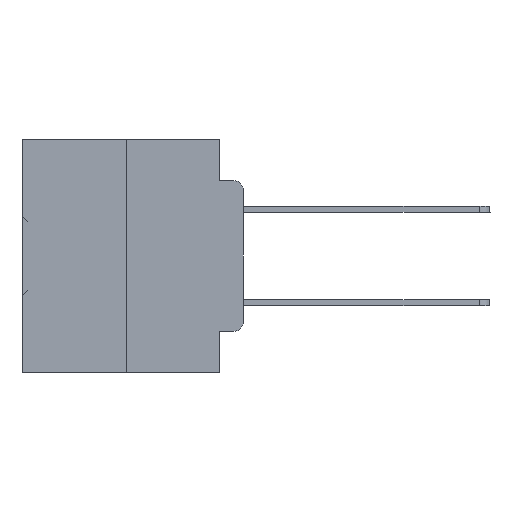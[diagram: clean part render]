
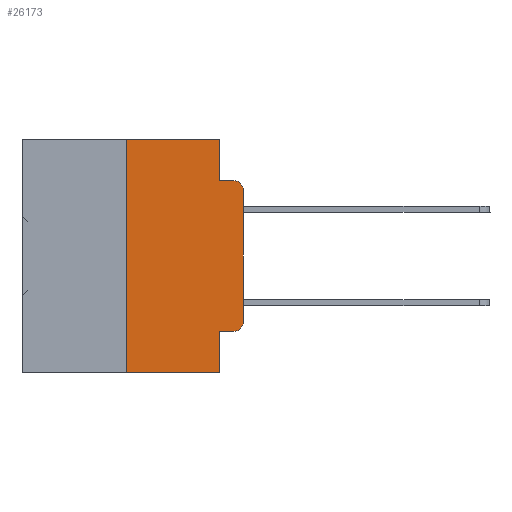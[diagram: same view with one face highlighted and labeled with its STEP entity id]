
A CAD part, left-side view. The second image highlights one B-rep face of the part: STEP entity #26173.
In plain terms, the highlighted planar face has unit normal (-1, 0, 0).
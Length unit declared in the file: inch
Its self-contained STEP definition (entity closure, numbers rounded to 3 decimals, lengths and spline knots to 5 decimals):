
#393 = FACE_OUTER_BOUND ( 'NONE', #2416, .T. ) ;
#561 = LINE ( 'NONE', #35942, #15969 ) ;
#688 = CARTESIAN_POINT ( 'NONE',  ( 0., 0.051, -0.4115 ) ) ;
#721 = EDGE_CURVE ( 'NONE', #11997, #14356, #5320, .T. ) ;
#747 = VERTEX_POINT ( 'NONE', #24021 ) ;
#1299 = DIRECTION ( 'NONE',  ( 0., -1., 0. ) ) ;
#1808 = DIRECTION ( 'NONE',  ( 0., 0., -1. ) ) ;
#2099 = LINE ( 'NONE', #9450, #25305 ) ;
#2406 = LINE ( 'NONE', #12970, #17697 ) ;
#2416 = EDGE_LOOP ( 'NONE', ( #24014, #24961, #5659, #21739, #38669, #31845, #33665, #26746, #3658, #13787 ) ) ;
#2659 = VERTEX_POINT ( 'NONE', #688 ) ;
#3182 = VERTEX_POINT ( 'NONE', #6799 ) ;
#3426 = VERTEX_POINT ( 'NONE', #30335 ) ;
#3658 = ORIENTED_EDGE ( 'NONE', *, *, #20122, .T. ) ;
#3841 = CIRCLE ( 'NONE', #37408, 0.02 ) ;
#4824 = LINE ( 'NONE', #29745, #35655 ) ;
#5126 = DIRECTION ( 'NONE',  ( 1., 0., 0. ) ) ;
#5320 = LINE ( 'NONE', #20551, #29268 ) ;
#5659 = ORIENTED_EDGE ( 'NONE', *, *, #33970, .F. ) ;
#6799 = CARTESIAN_POINT ( 'NONE',  ( 0., 0.25, 0. ) ) ;
#6877 = VERTEX_POINT ( 'NONE', #36498 ) ;
#7035 = CARTESIAN_POINT ( 'NONE',  ( 0., 0., -0.1085 ) ) ;
#7409 = CARTESIAN_POINT ( 'NONE',  ( 0., 0.25, -0.5 ) ) ;
#7493 = CIRCLE ( 'NONE', #21667, 0.02 ) ;
#8132 = LINE ( 'NONE', #19846, #14336 ) ;
#9295 = EDGE_CURVE ( 'NONE', #747, #32645, #2099, .T. ) ;
#9319 = DIRECTION ( 'NONE',  ( 0., 0., 1. ) ) ;
#9450 = CARTESIAN_POINT ( 'NONE',  ( 0., 0., 0. ) ) ;
#10491 = DIRECTION ( 'NONE',  ( 0., -1., 0. ) ) ;
#11108 = DIRECTION ( 'NONE',  ( -1., 0., 0. ) ) ;
#11997 = VERTEX_POINT ( 'NONE', #7409 ) ;
#12260 = VECTOR ( 'NONE', #1299, 39.37008 ) ;
#12970 = CARTESIAN_POINT ( 'NONE',  ( 0., 0.051, 0. ) ) ;
#13787 = ORIENTED_EDGE ( 'NONE', *, *, #18120, .T. ) ;
#14336 = VECTOR ( 'NONE', #22830, 39.37008 ) ;
#14356 = VERTEX_POINT ( 'NONE', #35133 ) ;
#14873 = VERTEX_POINT ( 'NONE', #37246 ) ;
#15969 = VECTOR ( 'NONE', #18272, 39.37008 ) ;
#15975 = DIRECTION ( 'NONE',  ( 0., 0., -1. ) ) ;
#16295 = VECTOR ( 'NONE', #10491, 39.37008 ) ;
#17183 = DIRECTION ( 'NONE',  ( 0., -1., 0. ) ) ;
#17697 = VECTOR ( 'NONE', #15975, 39.37008 ) ;
#18114 = AXIS2_PLACEMENT_3D ( 'NONE', #23183, #5126, #26160 ) ;
#18120 = EDGE_CURVE ( 'NONE', #3426, #747, #3841, .T. ) ;
#18272 = DIRECTION ( 'NONE',  ( 0., 0., 1. ) ) ;
#19080 = VERTEX_POINT ( 'NONE', #29603 ) ;
#19846 = CARTESIAN_POINT ( 'NONE',  ( 0., 0.473, 0. ) ) ;
#20054 = DIRECTION ( 'NONE',  ( -1., 0., 0. ) ) ;
#20122 = EDGE_CURVE ( 'NONE', #2659, #3426, #34964, .T. ) ;
#20551 = CARTESIAN_POINT ( 'NONE',  ( 0., 0.473, -0.5 ) ) ;
#21667 = AXIS2_PLACEMENT_3D ( 'NONE', #37681, #20054, #1808 ) ;
#21739 = ORIENTED_EDGE ( 'NONE', *, *, #32020, .F. ) ;
#22138 = EDGE_CURVE ( 'NONE', #2659, #14356, #4824, .T. ) ;
#22570 = CARTESIAN_POINT ( 'NONE',  ( 0., 0.051, -0.4115 ) ) ;
#22830 = DIRECTION ( 'NONE',  ( 0., -1., 0. ) ) ;
#23183 = CARTESIAN_POINT ( 'NONE',  ( 0., 0.473, 0. ) ) ;
#24014 = ORIENTED_EDGE ( 'NONE', *, *, #9295, .T. ) ;
#24021 = CARTESIAN_POINT ( 'NONE',  ( 0., 0., -0.3915 ) ) ;
#24961 = ORIENTED_EDGE ( 'NONE', *, *, #37881, .T. ) ;
#25305 = VECTOR ( 'NONE', #9319, 39.37008 ) ;
#26160 = DIRECTION ( 'NONE',  ( 0., 0., -1. ) ) ;
#26173 = ADVANCED_FACE ( 'NONE', ( #393 ), #37828, .F. ) ;
#26746 = ORIENTED_EDGE ( 'NONE', *, *, #22138, .F. ) ;
#28918 = CARTESIAN_POINT ( 'NONE',  ( 0., 0.02, -0.3915 ) ) ;
#29268 = VECTOR ( 'NONE', #17183, 39.37008 ) ;
#29271 = LINE ( 'NONE', #31315, #16295 ) ;
#29603 = CARTESIAN_POINT ( 'NONE',  ( 0., 0.051, -0.0885 ) ) ;
#29745 = CARTESIAN_POINT ( 'NONE',  ( 0., 0.051, 0. ) ) ;
#30033 = EDGE_CURVE ( 'NONE', #11997, #3182, #561, .T. ) ;
#30335 = CARTESIAN_POINT ( 'NONE',  ( 0., 0.02, -0.4115 ) ) ;
#31315 = CARTESIAN_POINT ( 'NONE',  ( 0., 0.051, -0.0885 ) ) ;
#31845 = ORIENTED_EDGE ( 'NONE', *, *, #30033, .F. ) ;
#31905 = DIRECTION ( 'NONE',  ( 0., 0., -1. ) ) ;
#32020 = EDGE_CURVE ( 'NONE', #6877, #19080, #2406, .T. ) ;
#32645 = VERTEX_POINT ( 'NONE', #7035 ) ;
#32696 = DIRECTION ( 'NONE',  ( 0., 0., -1. ) ) ;
#33665 = ORIENTED_EDGE ( 'NONE', *, *, #721, .T. ) ;
#33970 = EDGE_CURVE ( 'NONE', #19080, #14873, #29271, .T. ) ;
#34964 = LINE ( 'NONE', #22570, #12260 ) ;
#35133 = CARTESIAN_POINT ( 'NONE',  ( 0., 0.051, -0.5 ) ) ;
#35265 = EDGE_CURVE ( 'NONE', #3182, #6877, #8132, .T. ) ;
#35655 = VECTOR ( 'NONE', #32696, 39.37008 ) ;
#35942 = CARTESIAN_POINT ( 'NONE',  ( 0., 0.25, 0. ) ) ;
#36498 = CARTESIAN_POINT ( 'NONE',  ( 0., 0.051, 0. ) ) ;
#37246 = CARTESIAN_POINT ( 'NONE',  ( 0., 0.02, -0.0885 ) ) ;
#37408 = AXIS2_PLACEMENT_3D ( 'NONE', #28918, #11108, #31905 ) ;
#37681 = CARTESIAN_POINT ( 'NONE',  ( 0., 0.02, -0.1085 ) ) ;
#37828 = PLANE ( 'NONE',  #18114 ) ;
#37881 = EDGE_CURVE ( 'NONE', #32645, #14873, #7493, .T. ) ;
#38669 = ORIENTED_EDGE ( 'NONE', *, *, #35265, .F. ) ;
